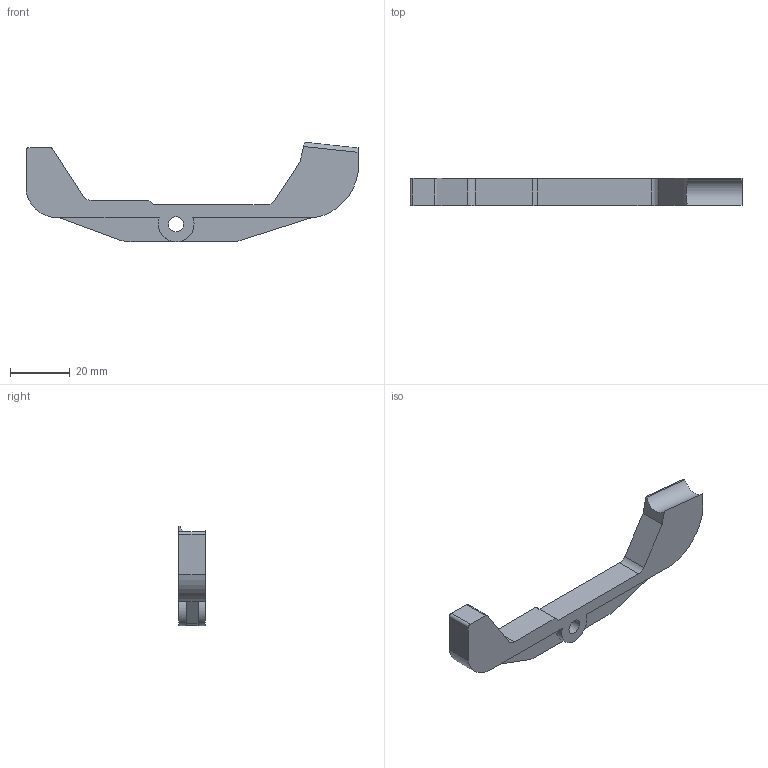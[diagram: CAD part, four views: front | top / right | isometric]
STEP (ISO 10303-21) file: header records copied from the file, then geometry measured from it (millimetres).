
FILE_DESCRIPTION (( 'STEP AP203' ), '1' );
FILE_NAME ('MOD9_ejector.STEP', '2020-06-10T04:58:07', ( '' ), ( '' ), 'SwSTEP 2.0', 'SolidWorks 2016', '' );
FILE_SCHEMA (( 'CONFIG_CONTROL_DESIGN' ));
Length unit declared in the file: millimetre
Products named in the file (1): MOD9_ejector
Bounding box: 111.36 x 9.05 x 33.39 mm (x, y, z)
Volume: 12368.4 mm3; surface area: 5999.2 mm2
Topology: 1 solids, 1 shells, 34 faces, 96 edges, 64 vertices
Faces by surface type: plane 23, cylinder 11
Full cylindrical faces by diameter (mm): 5.05 x1
Entity records: 1180 total; most frequent: CARTESIAN_POINT 200, ORIENTED_EDGE 190, DIRECTION 187, EDGE_CURVE 95, VECTOR 69, LINE 69, VERTEX_POINT 64, AXIS2_PLACEMENT_3D 59
